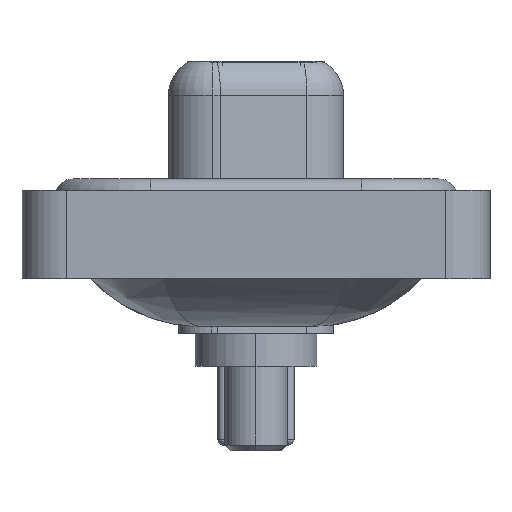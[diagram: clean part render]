
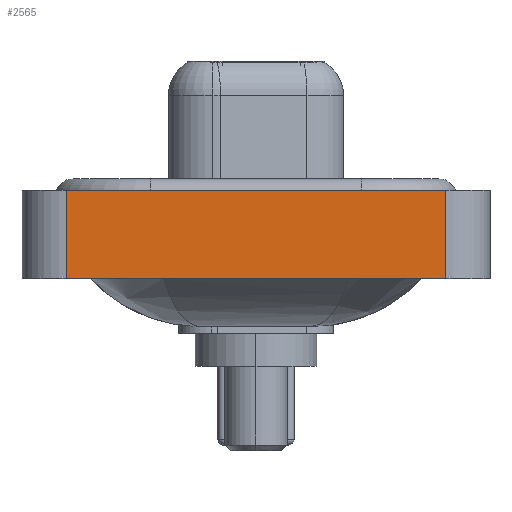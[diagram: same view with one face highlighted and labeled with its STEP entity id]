
A CAD part, left-side view. The second image highlights one B-rep face of the part: STEP entity #2565.
In plain terms, the highlighted planar face has unit normal (-1, 0, 0).
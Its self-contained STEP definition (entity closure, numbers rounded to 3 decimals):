
#578 = DIRECTION ( 'NONE',  ( -1., 0., 0. ) ) ;
#941 = VERTEX_POINT ( 'NONE', #19687 ) ;
#1103 = DIRECTION ( 'NONE',  ( 0., 0., 1. ) ) ;
#1923 = CARTESIAN_POINT ( 'NONE',  ( -7.3, -8.55, -3.6 ) ) ;
#1954 = EDGE_LOOP ( 'NONE', ( #10540, #14062, #1963, #20191 ) ) ;
#1963 = ORIENTED_EDGE ( 'NONE', *, *, #17692, .F. ) ;
#2565 = ADVANCED_FACE ( 'NONE', ( #11697 ), #17691, .T. ) ;
#2617 = LINE ( 'NONE', #2720, #10267 ) ;
#2720 = CARTESIAN_POINT ( 'NONE',  ( -7.3, -8.55, -3.6 ) ) ;
#4324 = EDGE_CURVE ( 'NONE', #13485, #11424, #19837, .T. ) ;
#4533 = EDGE_CURVE ( 'NONE', #10938, #11424, #19790, .T. ) ;
#5638 = DIRECTION ( 'NONE',  ( 0., -1., 0. ) ) ;
#5654 = DIRECTION ( 'NONE',  ( 0., 0., 1. ) ) ;
#7552 = CARTESIAN_POINT ( 'NONE',  ( -7.3, -8.55, -3.6 ) ) ;
#8464 = CARTESIAN_POINT ( 'NONE',  ( -7.3, -8.55, 0.4 ) ) ;
#8785 = LINE ( 'NONE', #18111, #12280 ) ;
#8792 = CARTESIAN_POINT ( 'NONE',  ( -7.3, -8.55, -3.6 ) ) ;
#9073 = DIRECTION ( 'NONE',  ( 0., -1., 0. ) ) ;
#9439 = EDGE_CURVE ( 'NONE', #941, #13485, #2617, .T. ) ;
#10267 = VECTOR ( 'NONE', #9073, 1000. ) ;
#10540 = ORIENTED_EDGE ( 'NONE', *, *, #4324, .T. ) ;
#10566 = VECTOR ( 'NONE', #1103, 1000. ) ;
#10938 = VERTEX_POINT ( 'NONE', #19882 ) ;
#11424 = VERTEX_POINT ( 'NONE', #14987 ) ;
#11697 = FACE_OUTER_BOUND ( 'NONE', #1954, .T. ) ;
#12280 = VECTOR ( 'NONE', #5654, 1000. ) ;
#13182 = AXIS2_PLACEMENT_3D ( 'NONE', #1923, #578, #13267 ) ;
#13267 = DIRECTION ( 'NONE',  ( 0., 0., 1. ) ) ;
#13485 = VERTEX_POINT ( 'NONE', #8792 ) ;
#14062 = ORIENTED_EDGE ( 'NONE', *, *, #4533, .F. ) ;
#14987 = CARTESIAN_POINT ( 'NONE',  ( -7.3, -8.55, 0.4 ) ) ;
#17691 = PLANE ( 'NONE',  #13182 ) ;
#17692 = EDGE_CURVE ( 'NONE', #941, #10938, #8785, .T. ) ;
#18111 = CARTESIAN_POINT ( 'NONE',  ( -7.3, 8.55, -3.6 ) ) ;
#19541 = VECTOR ( 'NONE', #5638, 1000. ) ;
#19687 = CARTESIAN_POINT ( 'NONE',  ( -7.3, 8.55, -3.6 ) ) ;
#19790 = LINE ( 'NONE', #8464, #19541 ) ;
#19837 = LINE ( 'NONE', #7552, #10566 ) ;
#19882 = CARTESIAN_POINT ( 'NONE',  ( -7.3, 8.55, 0.4 ) ) ;
#20191 = ORIENTED_EDGE ( 'NONE', *, *, #9439, .T. ) ;
